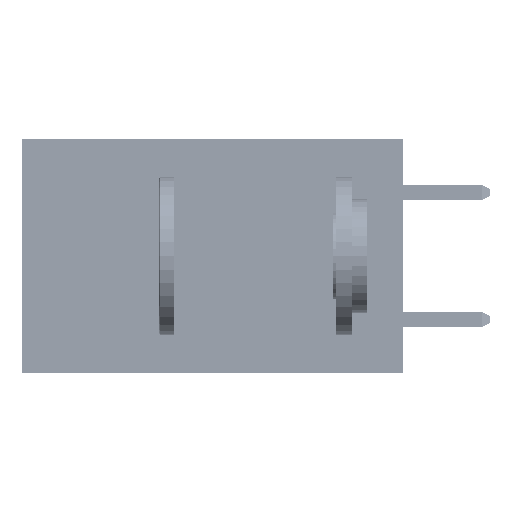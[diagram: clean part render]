
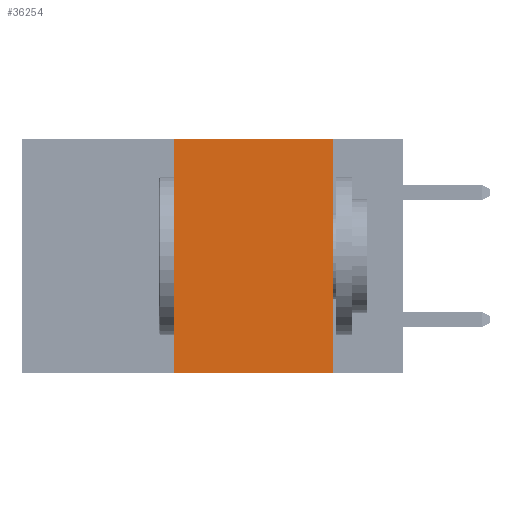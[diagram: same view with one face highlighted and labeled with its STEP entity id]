
A CAD part, left-side view. The second image highlights one B-rep face of the part: STEP entity #36254.
In plain terms, the highlighted planar face has unit normal (-1, 0, 0).
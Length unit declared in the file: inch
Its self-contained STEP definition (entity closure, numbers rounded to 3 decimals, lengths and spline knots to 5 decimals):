
#691 = LINE ( 'NONE', #16049, #39691 ) ;
#1119 = CARTESIAN_POINT ( 'NONE',  ( 0., 0.6, 0. ) ) ;
#1807 = CARTESIAN_POINT ( 'NONE',  ( 0., 0.6, 0. ) ) ;
#4427 = VERTEX_POINT ( 'NONE', #33487 ) ;
#5496 = DIRECTION ( 'NONE',  ( 0., -1., 0. ) ) ;
#8078 = ORIENTED_EDGE ( 'NONE', *, *, #26423, .F. ) ;
#10284 = DIRECTION ( 'NONE',  ( 0., 0., -1. ) ) ;
#13421 = VECTOR ( 'NONE', #20672, 39.37008 ) ;
#16049 = CARTESIAN_POINT ( 'NONE',  ( 0., 0.6, -0.37 ) ) ;
#18141 = FACE_OUTER_BOUND ( 'NONE', #25120, .T. ) ;
#19407 = EDGE_CURVE ( 'NONE', #47907, #4427, #691, .T. ) ;
#20131 = DIRECTION ( 'NONE',  ( 0., -1., 0. ) ) ;
#20672 = DIRECTION ( 'NONE',  ( 0., 0., -1. ) ) ;
#21441 = AXIS2_PLACEMENT_3D ( 'NONE', #1807, #33868, #10284 ) ;
#21653 = CARTESIAN_POINT ( 'NONE',  ( 0., 0.36, 0. ) ) ;
#22035 = LINE ( 'NONE', #21653, #30197 ) ;
#25120 = EDGE_LOOP ( 'NONE', ( #28316, #38357, #8078, #51950 ) ) ;
#26423 = EDGE_CURVE ( 'NONE', #47907, #37644, #22035, .T. ) ;
#28316 = ORIENTED_EDGE ( 'NONE', *, *, #29327, .F. ) ;
#28707 = CARTESIAN_POINT ( 'NONE',  ( 0., 0.11, 0. ) ) ;
#29327 = EDGE_CURVE ( 'NONE', #29671, #4427, #34824, .T. ) ;
#29671 = VERTEX_POINT ( 'NONE', #34483 ) ;
#30197 = VECTOR ( 'NONE', #33245, 39.37008 ) ;
#32135 = VECTOR ( 'NONE', #5496, 39.37008 ) ;
#32567 = CARTESIAN_POINT ( 'NONE',  ( 0., 0.36, -0.37 ) ) ;
#33245 = DIRECTION ( 'NONE',  ( 0., 0., 1. ) ) ;
#33487 = CARTESIAN_POINT ( 'NONE',  ( 0., 0.11, -0.37 ) ) ;
#33868 = DIRECTION ( 'NONE',  ( 1., 0., 0. ) ) ;
#34483 = CARTESIAN_POINT ( 'NONE',  ( 0., 0.11, 0. ) ) ;
#34824 = LINE ( 'NONE', #28707, #13421 ) ;
#34872 = CARTESIAN_POINT ( 'NONE',  ( 0., 0.36, 0. ) ) ;
#36254 = ADVANCED_FACE ( 'NONE', ( #18141 ), #42073, .F. ) ;
#37644 = VERTEX_POINT ( 'NONE', #34872 ) ;
#38357 = ORIENTED_EDGE ( 'NONE', *, *, #51784, .F. ) ;
#39691 = VECTOR ( 'NONE', #20131, 39.37008 ) ;
#42073 = PLANE ( 'NONE',  #21441 ) ;
#47769 = LINE ( 'NONE', #1119, #32135 ) ;
#47907 = VERTEX_POINT ( 'NONE', #32567 ) ;
#51784 = EDGE_CURVE ( 'NONE', #37644, #29671, #47769, .T. ) ;
#51950 = ORIENTED_EDGE ( 'NONE', *, *, #19407, .T. ) ;
